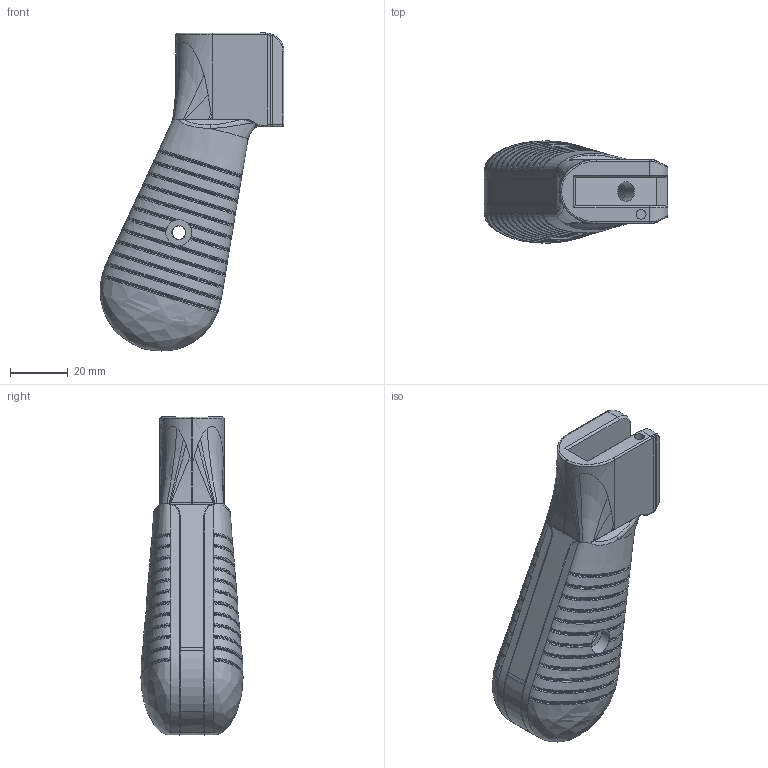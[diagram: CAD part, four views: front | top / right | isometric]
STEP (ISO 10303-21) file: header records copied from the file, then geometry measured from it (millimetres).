
FILE_DESCRIPTION(/* description */ (''),/* implementation_level */ '2;1');
FILE_NAME(/* name */ 'Final Concept.step',/* time_stamp */ '2021-09-21T09:20:59-04:00',/* author */ (''),/* organization */ (''),/* preprocessor_version */ 'ST-DEVELOPER v18.1',/* originating_system */ 'Autodesk Translation Framework v10.10.0.1391',/* authorisation */ '');
FILE_SCHEMA (('AUTOMOTIVE_DESIGN { 1 0 10303 214 3 1 1 }'));
Products named in the file (1): Final Concept
Bounding box: 63.48 x 35.27 x 109.89 mm (x, y, z)
Volume: 87160.8 mm3; surface area: 28907.7 mm2
Topology: 3 solids, 3 shells, 489 faces, 1217 edges, 741 vertices
Faces by surface type: bspline 242, plane 131, cylinder 69, torus 36, cone 11
Full cylindrical faces by diameter (mm): 3.4 x1, 4.6 x1, 4.8 x2, 6.8 x1, 9 x2, 13.165 x1
Entity records: 53639 total; most frequent: CARTESIAN_POINT 43780, ORIENTED_EDGE 2430, DIRECTION 1362, EDGE_CURVE 1215, VERTEX_POINT 741, B_SPLINE_CURVE_WITH_KNOTS 626, AXIS2_PLACEMENT_3D 525, EDGE_LOOP 514
